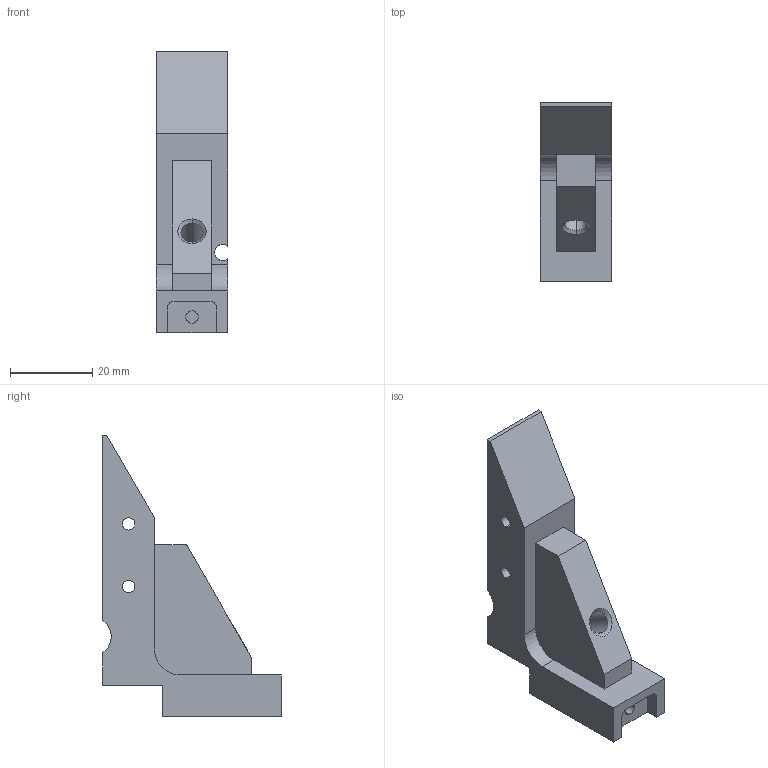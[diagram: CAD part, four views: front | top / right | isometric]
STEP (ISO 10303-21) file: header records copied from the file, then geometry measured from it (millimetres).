
FILE_DESCRIPTION (( 'STEP AP214' ), '1' );
FILE_NAME ('Reinforced_Grip_Part.step', '2015-06-12T17:08:57', ( '' ), ( '' ), 'SwSTEP 2.0', 'SolidWorks 2015', '' );
FILE_SCHEMA (( 'AUTOMOTIVE_DESIGN' ));
Length unit declared in the file: millimetre
Products named in the file (1): Reinforced_Grip_Part
Bounding box: 17.53 x 43.56 x 68.58 mm (x, y, z)
Volume: 18112.8 mm3; surface area: 8151.9 mm2
Topology: 1 solids, 1 shells, 69 faces, 193 edges, 128 vertices
Faces by surface type: plane 44, cylinder 23, cone 2
Entity records: 2312 total; most frequent: CARTESIAN_POINT 446, ORIENTED_EDGE 386, DIRECTION 370, EDGE_CURVE 193, LINE 142, VECTOR 142, VERTEX_POINT 128, AXIS2_PLACEMENT_3D 114
